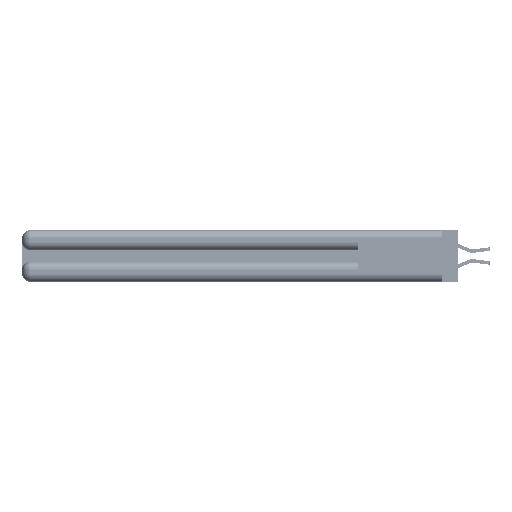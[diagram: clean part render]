
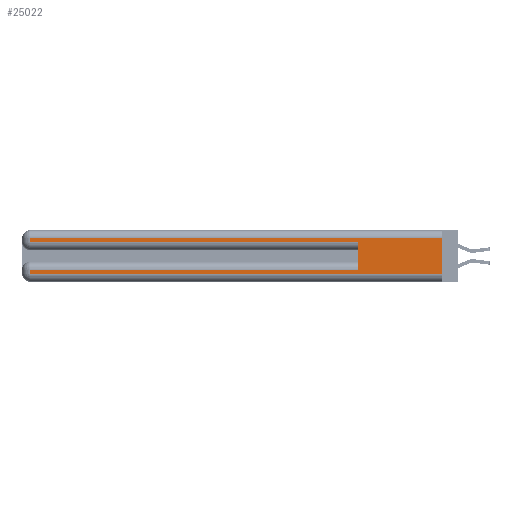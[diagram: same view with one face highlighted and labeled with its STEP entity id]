
A CAD part, left-side view. The second image highlights one B-rep face of the part: STEP entity #25022.
In plain terms, the highlighted planar face has unit normal (-1, 0, 0).
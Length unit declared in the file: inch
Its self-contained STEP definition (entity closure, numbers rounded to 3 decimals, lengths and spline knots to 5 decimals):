
#29 = ORIENTED_EDGE ( 'NONE', *, *, #29599, .F. ) ;
#181 = FACE_OUTER_BOUND ( 'NONE', #40426, .T. ) ;
#1469 = VECTOR ( 'NONE', #40469, 39.37008 ) ;
#2743 = CARTESIAN_POINT ( 'NONE',  ( 0., 2.94, 0.06 ) ) ;
#3139 = LINE ( 'NONE', #5515, #1469 ) ;
#3372 = CARTESIAN_POINT ( 'NONE',  ( 0., 0., 0.285 ) ) ;
#3393 = VERTEX_POINT ( 'NONE', #13463 ) ;
#3464 = DIRECTION ( 'NONE',  ( 0., 1., 0. ) ) ;
#4256 = CARTESIAN_POINT ( 'NONE',  ( 0., 0., 0.085 ) ) ;
#4679 = EDGE_CURVE ( 'NONE', #17944, #28147, #16185, .T. ) ;
#5073 = ORIENTED_EDGE ( 'NONE', *, *, #6005, .T. ) ;
#5515 = CARTESIAN_POINT ( 'NONE',  ( 0., 0., 0.06 ) ) ;
#6005 = EDGE_CURVE ( 'NONE', #3393, #17042, #38754, .T. ) ;
#6371 = LINE ( 'NONE', #3372, #17989 ) ;
#7963 = EDGE_CURVE ( 'NONE', #10753, #17944, #32421, .T. ) ;
#8651 = CARTESIAN_POINT ( 'NONE',  ( 0., 0., 0.37 ) ) ;
#9177 = ORIENTED_EDGE ( 'NONE', *, *, #4679, .T. ) ;
#9456 = DIRECTION ( 'NONE',  ( 0., 0., -1. ) ) ;
#10753 = VERTEX_POINT ( 'NONE', #33737 ) ;
#11907 = DIRECTION ( 'NONE',  ( 1., 0., 0. ) ) ;
#13169 = DIRECTION ( 'NONE',  ( 0., 0., 1. ) ) ;
#13463 = CARTESIAN_POINT ( 'NONE',  ( 0., 2.94, 0.085 ) ) ;
#14275 = VERTEX_POINT ( 'NONE', #18513 ) ;
#15602 = DIRECTION ( 'NONE',  ( 0., 1., 0. ) ) ;
#15850 = VECTOR ( 'NONE', #15602, 39.37008 ) ;
#16185 = LINE ( 'NONE', #38398, #44922 ) ;
#17042 = VERTEX_POINT ( 'NONE', #2743 ) ;
#17944 = VERTEX_POINT ( 'NONE', #39809 ) ;
#17989 = VECTOR ( 'NONE', #28093, 39.37008 ) ;
#18003 = DIRECTION ( 'NONE',  ( 0., 0., -1. ) ) ;
#18513 = CARTESIAN_POINT ( 'NONE',  ( 0., 0., 0.06 ) ) ;
#18712 = DIRECTION ( 'NONE',  ( 0., 0., -1. ) ) ;
#19133 = EDGE_CURVE ( 'NONE', #29699, #3393, #22969, .T. ) ;
#19345 = PLANE ( 'NONE',  #34503 ) ;
#20577 = CARTESIAN_POINT ( 'NONE',  ( 0., 0.6, 0.085 ) ) ;
#21074 = VECTOR ( 'NONE', #36786, 39.37008 ) ;
#21462 = ORIENTED_EDGE ( 'NONE', *, *, #19133, .T. ) ;
#21877 = LINE ( 'NONE', #30635, #39087 ) ;
#22969 = LINE ( 'NONE', #4256, #15850 ) ;
#25022 = ADVANCED_FACE ( 'NONE', ( #181 ), #19345, .F. ) ;
#28093 = DIRECTION ( 'NONE',  ( 0., -1., 0. ) ) ;
#28147 = VERTEX_POINT ( 'NONE', #44509 ) ;
#28844 = VERTEX_POINT ( 'NONE', #41221 ) ;
#28973 = VECTOR ( 'NONE', #13169, 39.37008 ) ;
#29599 = EDGE_CURVE ( 'NONE', #29699, #28844, #38950, .T. ) ;
#29699 = VERTEX_POINT ( 'NONE', #20577 ) ;
#30635 = CARTESIAN_POINT ( 'NONE',  ( 0., 0., 0.37 ) ) ;
#32283 = ORIENTED_EDGE ( 'NONE', *, *, #35609, .T. ) ;
#32300 = CARTESIAN_POINT ( 'NONE',  ( 0., 2.94, 0.37 ) ) ;
#32421 = LINE ( 'NONE', #34649, #42453 ) ;
#33737 = CARTESIAN_POINT ( 'NONE',  ( 0., 0., 0.31 ) ) ;
#34288 = CARTESIAN_POINT ( 'NONE',  ( 0., 0.6, 0.145 ) ) ;
#34503 = AXIS2_PLACEMENT_3D ( 'NONE', #8651, #11907, #18712 ) ;
#34649 = CARTESIAN_POINT ( 'NONE',  ( 0., 0., 0.31 ) ) ;
#35609 = EDGE_CURVE ( 'NONE', #17042, #14275, #3139, .T. ) ;
#36786 = DIRECTION ( 'NONE',  ( 0., 0., -1. ) ) ;
#38398 = CARTESIAN_POINT ( 'NONE',  ( 0., 2.94, 0.37 ) ) ;
#38754 = LINE ( 'NONE', #32300, #21074 ) ;
#38950 = LINE ( 'NONE', #34288, #28973 ) ;
#39087 = VECTOR ( 'NONE', #9456, 39.37008 ) ;
#39462 = ORIENTED_EDGE ( 'NONE', *, *, #7963, .T. ) ;
#39809 = CARTESIAN_POINT ( 'NONE',  ( 0., 2.94, 0.31 ) ) ;
#40426 = EDGE_LOOP ( 'NONE', ( #42858, #39462, #9177, #42256, #29, #21462, #5073, #32283 ) ) ;
#40469 = DIRECTION ( 'NONE',  ( 0., -1., 0. ) ) ;
#41221 = CARTESIAN_POINT ( 'NONE',  ( 0., 0.6, 0.285 ) ) ;
#42256 = ORIENTED_EDGE ( 'NONE', *, *, #44793, .T. ) ;
#42453 = VECTOR ( 'NONE', #3464, 39.37008 ) ;
#42858 = ORIENTED_EDGE ( 'NONE', *, *, #43865, .F. ) ;
#43865 = EDGE_CURVE ( 'NONE', #10753, #14275, #21877, .T. ) ;
#44509 = CARTESIAN_POINT ( 'NONE',  ( 0., 2.94, 0.285 ) ) ;
#44793 = EDGE_CURVE ( 'NONE', #28147, #28844, #6371, .T. ) ;
#44922 = VECTOR ( 'NONE', #18003, 39.37008 ) ;
